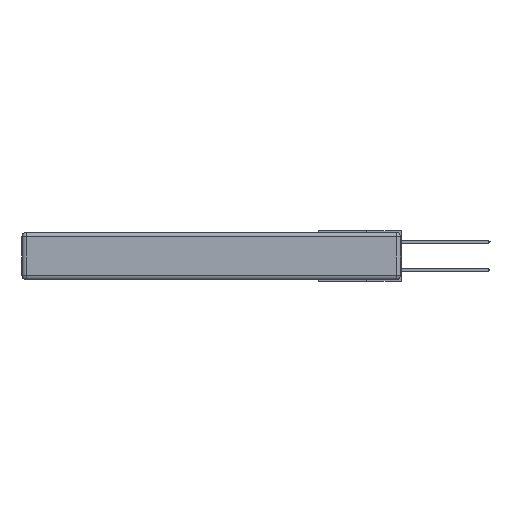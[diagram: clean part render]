
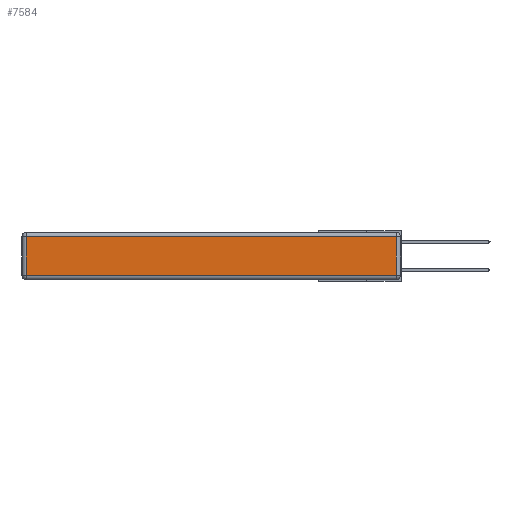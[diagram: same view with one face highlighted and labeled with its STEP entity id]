
A CAD part, left-side view. The second image highlights one B-rep face of the part: STEP entity #7584.
In plain terms, the highlighted planar face has unit normal (-1, 0, 0).
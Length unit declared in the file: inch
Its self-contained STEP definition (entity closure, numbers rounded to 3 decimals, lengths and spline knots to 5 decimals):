
#999 = CARTESIAN_POINT ( 'NONE',  ( 0., 0., -0.343 ) ) ;
#1417 = DIRECTION ( 'NONE',  ( 0., -1., 0. ) ) ;
#1445 = AXIS2_PLACEMENT_3D ( 'NONE', #999, #2911, #10338 ) ;
#1810 = LINE ( 'NONE', #21209, #11538 ) ;
#2911 = DIRECTION ( 'NONE',  ( -1., 0., 0. ) ) ;
#3348 = CARTESIAN_POINT ( 'NONE',  ( 0., 2.72, -0.313 ) ) ;
#3963 = ORIENTED_EDGE ( 'NONE', *, *, #8118, .T. ) ;
#4447 = VECTOR ( 'NONE', #1417, 39.37008 ) ;
#4790 = ORIENTED_EDGE ( 'NONE', *, *, #10111, .T. ) ;
#6370 = EDGE_CURVE ( 'NONE', #11111, #15994, #22804, .T. ) ;
#7546 = LINE ( 'NONE', #20798, #4447 ) ;
#7584 = ADVANCED_FACE ( 'NONE', ( #13536 ), #12253, .T. ) ;
#8118 = EDGE_CURVE ( 'NONE', #19017, #11111, #14346, .T. ) ;
#8122 = EDGE_CURVE ( 'NONE', #15994, #10298, #1810, .T. ) ;
#8202 = CARTESIAN_POINT ( 'NONE',  ( 0., 2.75, -0.03 ) ) ;
#8311 = CARTESIAN_POINT ( 'NONE',  ( 0., 2.72, -0.03 ) ) ;
#8767 = DIRECTION ( 'NONE',  ( 0., 0., 1. ) ) ;
#8867 = ORIENTED_EDGE ( 'NONE', *, *, #6370, .T. ) ;
#9997 = CARTESIAN_POINT ( 'NONE',  ( 0., 0.03, -0.313 ) ) ;
#10111 = EDGE_CURVE ( 'NONE', #10298, #19017, #7546, .T. ) ;
#10298 = VERTEX_POINT ( 'NONE', #3348 ) ;
#10338 = DIRECTION ( 'NONE',  ( 0., 0., 1. ) ) ;
#11111 = VERTEX_POINT ( 'NONE', #13925 ) ;
#11538 = VECTOR ( 'NONE', #14057, 39.37008 ) ;
#11762 = ORIENTED_EDGE ( 'NONE', *, *, #8122, .T. ) ;
#11823 = VECTOR ( 'NONE', #8767, 39.37008 ) ;
#12253 = PLANE ( 'NONE',  #1445 ) ;
#13536 = FACE_OUTER_BOUND ( 'NONE', #22089, .T. ) ;
#13925 = CARTESIAN_POINT ( 'NONE',  ( 0., 0.03, -0.03 ) ) ;
#14057 = DIRECTION ( 'NONE',  ( 0., 0., -1. ) ) ;
#14346 = LINE ( 'NONE', #19114, #11823 ) ;
#15534 = VECTOR ( 'NONE', #17455, 39.37008 ) ;
#15994 = VERTEX_POINT ( 'NONE', #8311 ) ;
#17455 = DIRECTION ( 'NONE',  ( 0., 1., 0. ) ) ;
#19017 = VERTEX_POINT ( 'NONE', #9997 ) ;
#19114 = CARTESIAN_POINT ( 'NONE',  ( 0., 0.03, -0.343 ) ) ;
#20798 = CARTESIAN_POINT ( 'NONE',  ( 0., 0., -0.313 ) ) ;
#21209 = CARTESIAN_POINT ( 'NONE',  ( 0., 2.72, -0.343 ) ) ;
#22089 = EDGE_LOOP ( 'NONE', ( #4790, #3963, #8867, #11762 ) ) ;
#22804 = LINE ( 'NONE', #8202, #15534 ) ;
